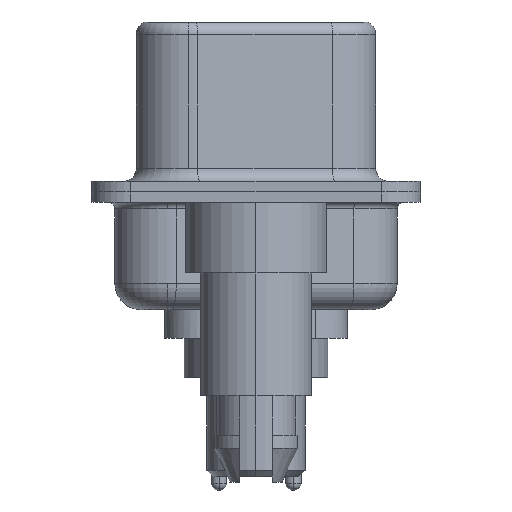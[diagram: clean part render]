
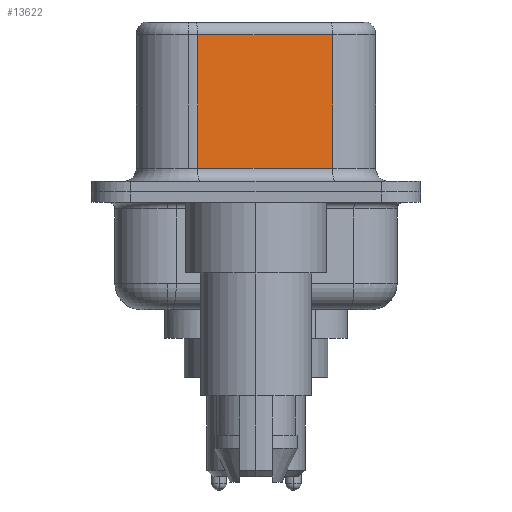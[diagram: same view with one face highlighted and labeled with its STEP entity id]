
A CAD part, left-side view. The second image highlights one B-rep face of the part: STEP entity #13622.
In plain terms, the highlighted planar face has unit normal (-0.985, -0.174, 0).
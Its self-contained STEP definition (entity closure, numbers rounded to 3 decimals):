
#168 = CARTESIAN_POINT ( 'NONE',  ( 3.655, 2.233, 6.52 ) ) ;
#721 = VERTEX_POINT ( 'NONE', #3386 ) ;
#1005 = CARTESIAN_POINT ( 'NONE',  ( 4.565, -2.927, 6.52 ) ) ;
#1420 = DIRECTION ( 'NONE',  ( 0., 0., -1. ) ) ;
#1736 = EDGE_CURVE ( 'NONE', #3174, #10702, #15796, .T. ) ;
#2154 = DIRECTION ( 'NONE',  ( 0., 0., -1. ) ) ;
#2396 = LINE ( 'NONE', #1005, #15574 ) ;
#2715 = CARTESIAN_POINT ( 'NONE',  ( 4.565, -2.927, 0.9 ) ) ;
#2946 = CARTESIAN_POINT ( 'NONE',  ( 3.655, 2.233, 6.02 ) ) ;
#3174 = VERTEX_POINT ( 'NONE', #11412 ) ;
#3386 = CARTESIAN_POINT ( 'NONE',  ( 4.565, -2.927, 6.02 ) ) ;
#4220 = VECTOR ( 'NONE', #12726, 1000. ) ;
#4342 = EDGE_CURVE ( 'NONE', #721, #10702, #2396, .T. ) ;
#4417 = VECTOR ( 'NONE', #1420, 1000. ) ;
#4454 = EDGE_CURVE ( 'NONE', #721, #9149, #7677, .T. ) ;
#5074 = DIRECTION ( 'NONE',  ( 0.174, -0.985, 0. ) ) ;
#6263 = EDGE_LOOP ( 'NONE', ( #11071, #10114, #13584, #10944 ) ) ;
#6958 = CARTESIAN_POINT ( 'NONE',  ( 4.565, -2.927, 6.52 ) ) ;
#7677 = LINE ( 'NONE', #14684, #4220 ) ;
#8234 = DIRECTION ( 'NONE',  ( -0.174, 0.985, 0. ) ) ;
#9149 = VERTEX_POINT ( 'NONE', #2946 ) ;
#9250 = CARTESIAN_POINT ( 'NONE',  ( 4.565, -2.927, 0.9 ) ) ;
#9535 = AXIS2_PLACEMENT_3D ( 'NONE', #6958, #15832, #8234 ) ;
#10114 = ORIENTED_EDGE ( 'NONE', *, *, #4454, .T. ) ;
#10702 = VERTEX_POINT ( 'NONE', #9250 ) ;
#10944 = ORIENTED_EDGE ( 'NONE', *, *, #1736, .T. ) ;
#11071 = ORIENTED_EDGE ( 'NONE', *, *, #4342, .F. ) ;
#11195 = LINE ( 'NONE', #168, #4417 ) ;
#11412 = CARTESIAN_POINT ( 'NONE',  ( 3.655, 2.233, 0.9 ) ) ;
#12374 = VECTOR ( 'NONE', #5074, 1000. ) ;
#12726 = DIRECTION ( 'NONE',  ( -0.174, 0.985, 0. ) ) ;
#13367 = FACE_OUTER_BOUND ( 'NONE', #6263, .T. ) ;
#13584 = ORIENTED_EDGE ( 'NONE', *, *, #14778, .T. ) ;
#13622 = ADVANCED_FACE ( 'NONE', ( #13367 ), #14536, .F. ) ;
#14536 = PLANE ( 'NONE',  #9535 ) ;
#14684 = CARTESIAN_POINT ( 'NONE',  ( 4.565, -2.927, 6.02 ) ) ;
#14778 = EDGE_CURVE ( 'NONE', #9149, #3174, #11195, .T. ) ;
#15574 = VECTOR ( 'NONE', #2154, 1000. ) ;
#15796 = LINE ( 'NONE', #2715, #12374 ) ;
#15832 = DIRECTION ( 'NONE',  ( 0.985, 0.174, 0. ) ) ;
